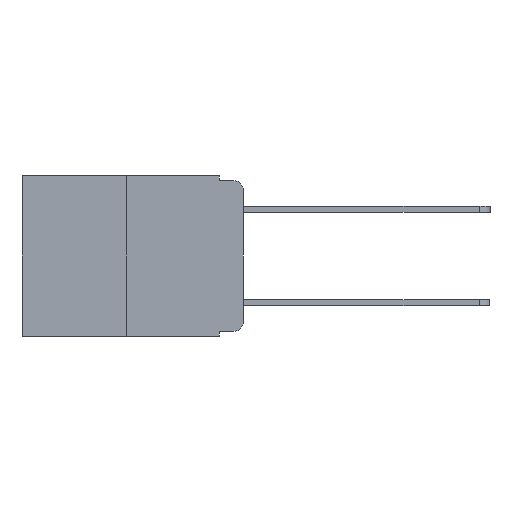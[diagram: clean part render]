
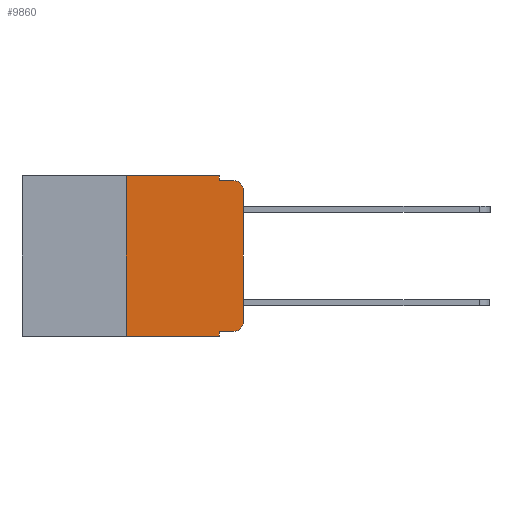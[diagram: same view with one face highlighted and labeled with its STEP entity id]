
A CAD part, left-side view. The second image highlights one B-rep face of the part: STEP entity #9860.
In plain terms, the highlighted planar face has unit normal (-1, 0, 0).
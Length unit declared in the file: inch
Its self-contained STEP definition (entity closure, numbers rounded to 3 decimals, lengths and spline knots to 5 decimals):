
#65 = ORIENTED_EDGE ( 'NONE', *, *, #3939, .T. ) ;
#105 = VECTOR ( 'NONE', #6703, 39.37008 ) ;
#580 = CARTESIAN_POINT ( 'NONE',  ( 0., 0.25, 0. ) ) ;
#652 = VERTEX_POINT ( 'NONE', #12319 ) ;
#670 = ORIENTED_EDGE ( 'NONE', *, *, #5267, .F. ) ;
#904 = EDGE_CURVE ( 'NONE', #652, #2123, #14745, .T. ) ;
#1538 = VECTOR ( 'NONE', #16213, 39.37008 ) ;
#1985 = EDGE_CURVE ( 'NONE', #9336, #652, #11233, .T. ) ;
#2038 = CARTESIAN_POINT ( 'NONE',  ( 0., 0.25, -0.343 ) ) ;
#2123 = VERTEX_POINT ( 'NONE', #12964 ) ;
#2206 = LINE ( 'NONE', #9105, #8442 ) ;
#2439 = CARTESIAN_POINT ( 'NONE',  ( 0., 0.02, -0.333 ) ) ;
#2496 = CARTESIAN_POINT ( 'NONE',  ( 0., 0.051, -0.343 ) ) ;
#2745 = DIRECTION ( 'NONE',  ( 0., -1., 0. ) ) ;
#2979 = CIRCLE ( 'NONE', #14252, 0.02 ) ;
#3022 = AXIS2_PLACEMENT_3D ( 'NONE', #12746, #12640, #12489 ) ;
#3135 = CARTESIAN_POINT ( 'NONE',  ( 0., 0.051, -0.01 ) ) ;
#3214 = ORIENTED_EDGE ( 'NONE', *, *, #904, .F. ) ;
#3754 = VECTOR ( 'NONE', #14851, 39.37008 ) ;
#3776 = CARTESIAN_POINT ( 'NONE',  ( 0., 0.051, -0.333 ) ) ;
#3939 = EDGE_CURVE ( 'NONE', #4146, #8609, #2206, .T. ) ;
#4146 = VERTEX_POINT ( 'NONE', #14022 ) ;
#4751 = EDGE_CURVE ( 'NONE', #8609, #10690, #12864, .T. ) ;
#4813 = ORIENTED_EDGE ( 'NONE', *, *, #7441, .T. ) ;
#5013 = DIRECTION ( 'NONE',  ( 0., 0., -1. ) ) ;
#5181 = ORIENTED_EDGE ( 'NONE', *, *, #14616, .F. ) ;
#5225 = FACE_OUTER_BOUND ( 'NONE', #5356, .T. ) ;
#5241 = CARTESIAN_POINT ( 'NONE',  ( 0., 0.473, -0.343 ) ) ;
#5267 = EDGE_CURVE ( 'NONE', #8946, #9336, #5922, .T. ) ;
#5356 = EDGE_LOOP ( 'NONE', ( #65, #8644, #5181, #3214, #12904, #670, #14774, #11936, #6951, #4813 ) ) ;
#5397 = DIRECTION ( 'NONE',  ( -1., 0., 0. ) ) ;
#5922 = LINE ( 'NONE', #580, #15609 ) ;
#6199 = VECTOR ( 'NONE', #2745, 39.37008 ) ;
#6323 = CARTESIAN_POINT ( 'NONE',  ( 0., 0.051, 0. ) ) ;
#6580 = LINE ( 'NONE', #5241, #6199 ) ;
#6639 = LINE ( 'NONE', #6323, #3754 ) ;
#6703 = DIRECTION ( 'NONE',  ( 0., -1., 0. ) ) ;
#6951 = ORIENTED_EDGE ( 'NONE', *, *, #12699, .T. ) ;
#7240 = VERTEX_POINT ( 'NONE', #2439 ) ;
#7259 = VERTEX_POINT ( 'NONE', #2496 ) ;
#7441 = EDGE_CURVE ( 'NONE', #7240, #4146, #2979, .T. ) ;
#7699 = AXIS2_PLACEMENT_3D ( 'NONE', #9946, #12406, #5013 ) ;
#7751 = VECTOR ( 'NONE', #12980, 39.37008 ) ;
#8442 = VECTOR ( 'NONE', #13924, 39.37008 ) ;
#8561 = EDGE_CURVE ( 'NONE', #11403, #7259, #6639, .T. ) ;
#8609 = VERTEX_POINT ( 'NONE', #11320 ) ;
#8644 = ORIENTED_EDGE ( 'NONE', *, *, #4751, .T. ) ;
#8946 = VERTEX_POINT ( 'NONE', #2038 ) ;
#9066 = CARTESIAN_POINT ( 'NONE',  ( 0., 0.25, 0. ) ) ;
#9105 = CARTESIAN_POINT ( 'NONE',  ( 0., 0., 0. ) ) ;
#9336 = VERTEX_POINT ( 'NONE', #9066 ) ;
#9860 = ADVANCED_FACE ( 'NONE', ( #5225 ), #14767, .F. ) ;
#9946 = CARTESIAN_POINT ( 'NONE',  ( 0., 0.473, 0. ) ) ;
#10690 = VERTEX_POINT ( 'NONE', #13919 ) ;
#10832 = VECTOR ( 'NONE', #11929, 39.37008 ) ;
#11035 = LINE ( 'NONE', #3135, #7751 ) ;
#11233 = LINE ( 'NONE', #13759, #10832 ) ;
#11320 = CARTESIAN_POINT ( 'NONE',  ( 0., 0., -0.03 ) ) ;
#11403 = VERTEX_POINT ( 'NONE', #3776 ) ;
#11929 = DIRECTION ( 'NONE',  ( 0., -1., 0. ) ) ;
#11936 = ORIENTED_EDGE ( 'NONE', *, *, #8561, .F. ) ;
#12319 = CARTESIAN_POINT ( 'NONE',  ( 0., 0.051, 0. ) ) ;
#12406 = DIRECTION ( 'NONE',  ( 1., 0., 0. ) ) ;
#12489 = DIRECTION ( 'NONE',  ( 0., 0., -1. ) ) ;
#12640 = DIRECTION ( 'NONE',  ( -1., 0., 0. ) ) ;
#12699 = EDGE_CURVE ( 'NONE', #11403, #7240, #13239, .T. ) ;
#12746 = CARTESIAN_POINT ( 'NONE',  ( 0., 0.02, -0.03 ) ) ;
#12770 = CARTESIAN_POINT ( 'NONE',  ( 0., 0.02, -0.313 ) ) ;
#12864 = CIRCLE ( 'NONE', #3022, 0.02 ) ;
#12904 = ORIENTED_EDGE ( 'NONE', *, *, #1985, .F. ) ;
#12964 = CARTESIAN_POINT ( 'NONE',  ( 0., 0.051, -0.01 ) ) ;
#12980 = DIRECTION ( 'NONE',  ( 0., -1., 0. ) ) ;
#13179 = DIRECTION ( 'NONE',  ( 0., 0., 1. ) ) ;
#13239 = LINE ( 'NONE', #14044, #105 ) ;
#13759 = CARTESIAN_POINT ( 'NONE',  ( 0., 0.473, 0. ) ) ;
#13919 = CARTESIAN_POINT ( 'NONE',  ( 0., 0.02, -0.01 ) ) ;
#13924 = DIRECTION ( 'NONE',  ( 0., 0., 1. ) ) ;
#13992 = DIRECTION ( 'NONE',  ( 0., 0., -1. ) ) ;
#14022 = CARTESIAN_POINT ( 'NONE',  ( 0., 0., -0.313 ) ) ;
#14044 = CARTESIAN_POINT ( 'NONE',  ( 0., 0.051, -0.333 ) ) ;
#14252 = AXIS2_PLACEMENT_3D ( 'NONE', #12770, #5397, #13992 ) ;
#14616 = EDGE_CURVE ( 'NONE', #2123, #10690, #11035, .T. ) ;
#14745 = LINE ( 'NONE', #15440, #1538 ) ;
#14767 = PLANE ( 'NONE',  #7699 ) ;
#14774 = ORIENTED_EDGE ( 'NONE', *, *, #15659, .T. ) ;
#14851 = DIRECTION ( 'NONE',  ( 0., 0., -1. ) ) ;
#15440 = CARTESIAN_POINT ( 'NONE',  ( 0., 0.051, 0. ) ) ;
#15609 = VECTOR ( 'NONE', #13179, 39.37008 ) ;
#15659 = EDGE_CURVE ( 'NONE', #8946, #7259, #6580, .T. ) ;
#16213 = DIRECTION ( 'NONE',  ( 0., 0., -1. ) ) ;
